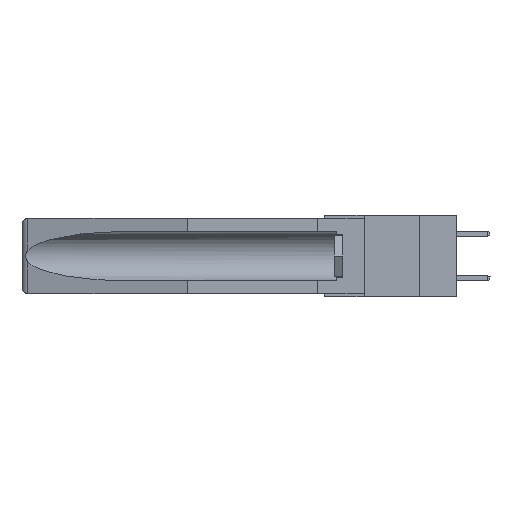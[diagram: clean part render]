
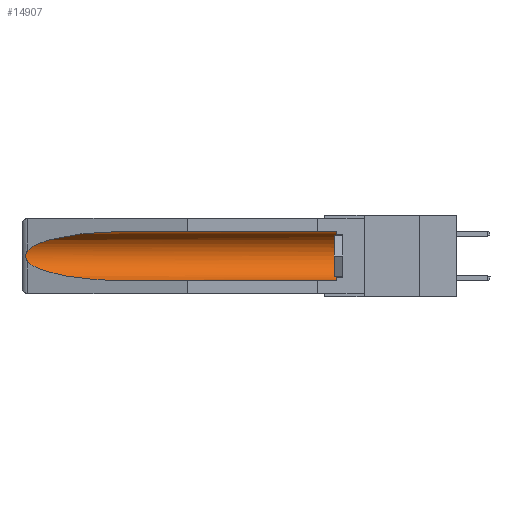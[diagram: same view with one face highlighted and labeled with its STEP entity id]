
A CAD part, left-side view. The second image highlights one B-rep face of the part: STEP entity #14907.
In plain terms, the highlighted cylindrical face has radius 2.857 mm (diameter 5.715 mm), a partial arc.
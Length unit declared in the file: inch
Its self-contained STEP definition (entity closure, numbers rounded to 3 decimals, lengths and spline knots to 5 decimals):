
#15 = CARTESIAN_POINT ( 'NONE',  ( 0.155, -0.30754, -0.1715 ) ) ;
#130 = VECTOR ( 'NONE', #10463, 39.37008 ) ;
#187 = VERTEX_POINT ( 'NONE', #13854 ) ;
#191 = CIRCLE ( 'NONE', #12109, 0.1125 ) ;
#193 = CARTESIAN_POINT ( 'NONE',  ( 0.155, 1.07973, -0.059 ) ) ;
#861 = ORIENTED_EDGE ( 'NONE', *, *, #3214, .T. ) ;
#1478 = CARTESIAN_POINT ( 'NONE',  ( 0.26537, 1.52718, -0.14972 ) ) ;
#1564 = DIRECTION ( 'NONE',  ( 0., -1., 0. ) ) ;
#1715 = CARTESIAN_POINT ( 'NONE',  ( 0.26597, 1.5296, -0.19026 ) ) ;
#1897 = CARTESIAN_POINT ( 'NONE',  ( 0.26597, 1.52961, -0.15275 ) ) ;
#1929 = B_SPLINE_CURVE_WITH_KNOTS ( 'NONE', 3,
 ( #5680, #1897, #15025, #14070, #8845, #8900, #2538, #14012, #1715, #2865 ),
 .UNSPECIFIED., .F., .F.,
 ( 4, 2, 2, 2, 4 ),
 ( 0., 0.00029, 0.00058, 0.00087, 0.00117 ),
 .UNSPECIFIED. ) ;
#2075 = CARTESIAN_POINT ( 'NONE',  ( 0.25451, 1.48313, -0.24835 ) ) ;
#2538 = CARTESIAN_POINT ( 'NONE',  ( 0.2673, 1.53269, -0.17917 ) ) ;
#2865 = CARTESIAN_POINT ( 'NONE',  ( 0.26537, 1.52718, -0.19328 ) ) ;
#2927 = FACE_OUTER_BOUND ( 'NONE', #10294, .T. ) ;
#3214 = EDGE_CURVE ( 'NONE', #14317, #187, #191, .T. ) ;
#3292 = CARTESIAN_POINT ( 'NONE',  ( 0.155, 1.07973, -0.284 ) ) ;
#3408 = CARTESIAN_POINT ( 'NONE',  ( 0.21114, 1.30732, -0.284 ) ) ;
#3533 = LINE ( 'NONE', #13021, #130 ) ;
#3770 = DIRECTION ( 'NONE',  ( 0., 1., 0. ) ) ;
#4139 = CARTESIAN_POINT ( 'NONE',  ( 0.25451, 1.48313, -0.09465 ) ) ;
#4531 = EDGE_CURVE ( 'NONE', #6967, #5820, #8863, .T. ) ;
#4760 = ORIENTED_EDGE ( 'NONE', *, *, #4531, .T. ) ;
#4929 = EDGE_CURVE ( 'NONE', #187, #6967, #3533, .T. ) ;
#5172 = ORIENTED_EDGE ( 'NONE', *, *, #6691, .F. ) ;
#5502 = DIRECTION ( 'NONE',  ( 0., 0., 1. ) ) ;
#5680 = CARTESIAN_POINT ( 'NONE',  ( 0.26537, 1.52718, -0.14972 ) ) ;
#5820 = VERTEX_POINT ( 'NONE', #7924 ) ;
#6072 = VECTOR ( 'NONE', #11432, 39.37008 ) ;
#6261 = ORIENTED_EDGE ( 'NONE', *, *, #14642, .T. ) ;
#6315 = CYLINDRICAL_SURFACE ( 'NONE', #6627, 0.1125 ) ;
#6627 = AXIS2_PLACEMENT_3D ( 'NONE', #15, #3770, #7630 ) ;
#6691 = EDGE_CURVE ( 'NONE', #14317, #11809, #9671, .T. ) ;
#6752 = ORIENTED_EDGE ( 'NONE', *, *, #4929, .T. ) ;
#6967 = VERTEX_POINT ( 'NONE', #14929 ) ;
#7115 = CARTESIAN_POINT ( 'NONE',  ( 0.26537, 1.52718, -0.19328 ) ) ;
#7630 = DIRECTION ( 'NONE',  ( 0., 0., 1. ) ) ;
#7924 = CARTESIAN_POINT ( 'NONE',  ( 0.26537, 1.52718, -0.14972 ) ) ;
#8845 = CARTESIAN_POINT ( 'NONE',  ( 0.2675, 1.53308, -0.16763 ) ) ;
#8863 =( BOUNDED_CURVE ( )  B_SPLINE_CURVE ( 3, ( #193, #9330, #4139, #1478 ),
 .UNSPECIFIED., .F., .F. ) 
 B_SPLINE_CURVE_WITH_KNOTS ( ( 4, 4 ),
 ( 4.71239, 6.08839 ),
 .UNSPECIFIED. ) 
 CURVE ( )  GEOMETRIC_REPRESENTATION_ITEM ( )  RATIONAL_B_SPLINE_CURVE ( ( 1., 0.848, 0.848, 1. ) ) 
 REPRESENTATION_ITEM ( '' )  );
#8900 = CARTESIAN_POINT ( 'NONE',  ( 0.2675, 1.53308, -0.17534 ) ) ;
#8950 = CARTESIAN_POINT ( 'NONE',  ( 0.155, -0.30754, -0.284 ) ) ;
#9330 = CARTESIAN_POINT ( 'NONE',  ( 0.21114, 1.30732, -0.059 ) ) ;
#9671 = LINE ( 'NONE', #8950, #6072 ) ;
#9732 = EDGE_CURVE ( 'NONE', #5820, #12907, #1929, .T. ) ;
#10294 = EDGE_LOOP ( 'NONE', ( #4760, #15729, #6261, #5172, #861, #6752 ) ) ;
#10463 = DIRECTION ( 'NONE',  ( 0., 1., 0. ) ) ;
#11432 = DIRECTION ( 'NONE',  ( 0., 1., 0. ) ) ;
#11809 = VERTEX_POINT ( 'NONE', #16388 ) ;
#11882 = CARTESIAN_POINT ( 'NONE',  ( 0.155, 0.126, -0.1715 ) ) ;
#12109 = AXIS2_PLACEMENT_3D ( 'NONE', #11882, #1564, #5502 ) ;
#12907 = VERTEX_POINT ( 'NONE', #7115 ) ;
#13021 = CARTESIAN_POINT ( 'NONE',  ( 0.155, -0.30754, -0.059 ) ) ;
#13854 = CARTESIAN_POINT ( 'NONE',  ( 0.155, 0.126, -0.059 ) ) ;
#14012 = CARTESIAN_POINT ( 'NONE',  ( 0.26655, 1.53094, -0.18657 ) ) ;
#14070 = CARTESIAN_POINT ( 'NONE',  ( 0.2673, 1.5327, -0.16383 ) ) ;
#14317 = VERTEX_POINT ( 'NONE', #14372 ) ;
#14357 =( BOUNDED_CURVE ( )  B_SPLINE_CURVE ( 3, ( #16186, #2075, #3408, #3292 ),
 .UNSPECIFIED., .F., .F. ) 
 B_SPLINE_CURVE_WITH_KNOTS ( ( 4, 4 ),
 ( 0.1948, 1.5708 ),
 .UNSPECIFIED. ) 
 CURVE ( )  GEOMETRIC_REPRESENTATION_ITEM ( )  RATIONAL_B_SPLINE_CURVE ( ( 1., 0.848, 0.848, 1. ) ) 
 REPRESENTATION_ITEM ( '' )  );
#14372 = CARTESIAN_POINT ( 'NONE',  ( 0.155, 0.126, -0.284 ) ) ;
#14642 = EDGE_CURVE ( 'NONE', #12907, #11809, #14357, .T. ) ;
#14907 = ADVANCED_FACE ( 'NONE', ( #2927 ), #6315, .F. ) ;
#14929 = CARTESIAN_POINT ( 'NONE',  ( 0.155, 1.07973, -0.059 ) ) ;
#15025 = CARTESIAN_POINT ( 'NONE',  ( 0.26654, 1.53092, -0.15636 ) ) ;
#15729 = ORIENTED_EDGE ( 'NONE', *, *, #9732, .T. ) ;
#16186 = CARTESIAN_POINT ( 'NONE',  ( 0.26537, 1.52718, -0.19328 ) ) ;
#16388 = CARTESIAN_POINT ( 'NONE',  ( 0.155, 1.07973, -0.284 ) ) ;
